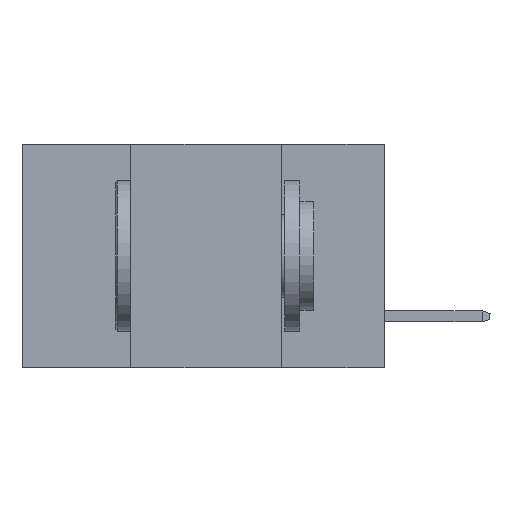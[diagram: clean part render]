
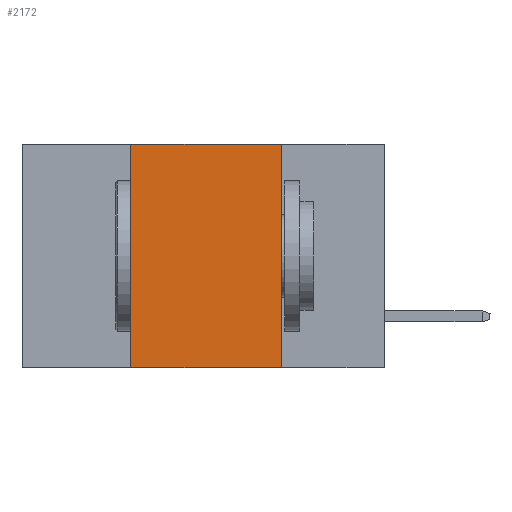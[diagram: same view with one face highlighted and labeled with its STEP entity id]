
A CAD part, left-side view. The second image highlights one B-rep face of the part: STEP entity #2172.
In plain terms, the highlighted planar face has unit normal (-1, 0, 0).
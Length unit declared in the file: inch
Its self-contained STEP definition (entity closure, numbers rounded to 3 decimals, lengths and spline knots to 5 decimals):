
#342 = FACE_OUTER_BOUND ( 'NONE', #24177, .T. ) ;
#1494 = DIRECTION ( 'NONE',  ( 0., -1., 0. ) ) ;
#1762 = CARTESIAN_POINT ( 'NONE',  ( 0., 0.6, 0. ) ) ;
#1933 = CARTESIAN_POINT ( 'NONE',  ( 0., 0.42, 0. ) ) ;
#2172 = ADVANCED_FACE ( 'NONE', ( #342 ), #13937, .F. ) ;
#3265 = CARTESIAN_POINT ( 'NONE',  ( 0., 0.42, -0.37 ) ) ;
#4509 = CARTESIAN_POINT ( 'NONE',  ( 0., 0.6, -0.37 ) ) ;
#6030 = DIRECTION ( 'NONE',  ( 0., 0., -1. ) ) ;
#6454 = LINE ( 'NONE', #3265, #23702 ) ;
#7008 = ORIENTED_EDGE ( 'NONE', *, *, #21814, .F. ) ;
#7447 = CARTESIAN_POINT ( 'NONE',  ( 0., 0.17, -0.37 ) ) ;
#8575 = LINE ( 'NONE', #4509, #24910 ) ;
#9755 = CARTESIAN_POINT ( 'NONE',  ( 0., 0.17, -0.37 ) ) ;
#13909 = AXIS2_PLACEMENT_3D ( 'NONE', #16054, #24097, #6030 ) ;
#13937 = PLANE ( 'NONE',  #13909 ) ;
#14327 = VERTEX_POINT ( 'NONE', #15559 ) ;
#14364 = CARTESIAN_POINT ( 'NONE',  ( 0., 0.42, -0.37 ) ) ;
#15559 = CARTESIAN_POINT ( 'NONE',  ( 0., 0.17, 0. ) ) ;
#15604 = VERTEX_POINT ( 'NONE', #1933 ) ;
#16054 = CARTESIAN_POINT ( 'NONE',  ( 0., 0.6, 0. ) ) ;
#16178 = ORIENTED_EDGE ( 'NONE', *, *, #16589, .T. ) ;
#16589 = EDGE_CURVE ( 'NONE', #24880, #17209, #8575, .T. ) ;
#17209 = VERTEX_POINT ( 'NONE', #7447 ) ;
#17576 = VECTOR ( 'NONE', #22029, 39.37008 ) ;
#18476 = EDGE_CURVE ( 'NONE', #24880, #15604, #6454, .T. ) ;
#19873 = ORIENTED_EDGE ( 'NONE', *, *, #24638, .F. ) ;
#20729 = DIRECTION ( 'NONE',  ( 0., -1., 0. ) ) ;
#21814 = EDGE_CURVE ( 'NONE', #15604, #14327, #23546, .T. ) ;
#22029 = DIRECTION ( 'NONE',  ( 0., 0., -1. ) ) ;
#22148 = VECTOR ( 'NONE', #1494, 39.37008 ) ;
#23076 = DIRECTION ( 'NONE',  ( 0., 0., 1. ) ) ;
#23546 = LINE ( 'NONE', #1762, #22148 ) ;
#23702 = VECTOR ( 'NONE', #23076, 39.37008 ) ;
#24097 = DIRECTION ( 'NONE',  ( 1., 0., 0. ) ) ;
#24177 = EDGE_LOOP ( 'NONE', ( #19873, #7008, #25726, #16178 ) ) ;
#24638 = EDGE_CURVE ( 'NONE', #14327, #17209, #25711, .T. ) ;
#24880 = VERTEX_POINT ( 'NONE', #14364 ) ;
#24910 = VECTOR ( 'NONE', #20729, 39.37008 ) ;
#25711 = LINE ( 'NONE', #9755, #17576 ) ;
#25726 = ORIENTED_EDGE ( 'NONE', *, *, #18476, .F. ) ;
